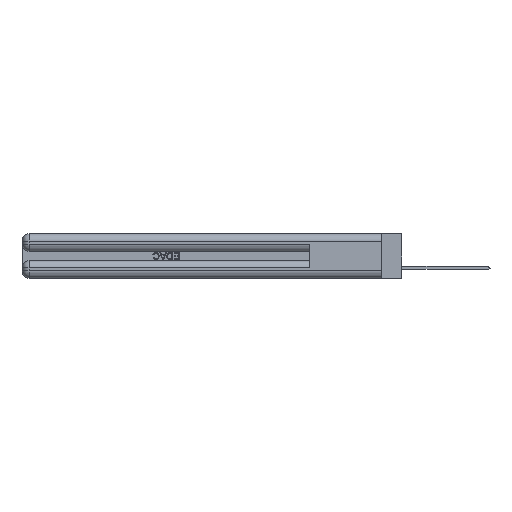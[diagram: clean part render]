
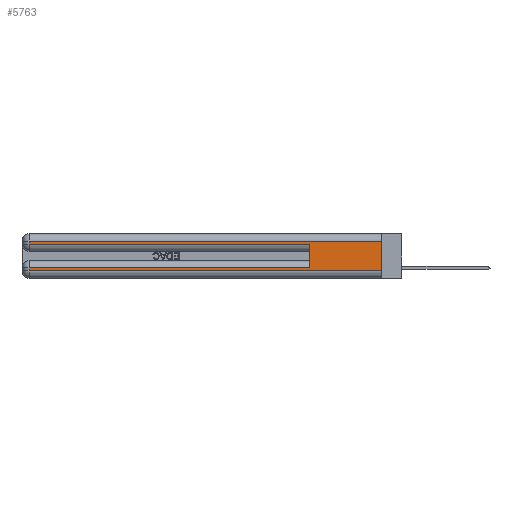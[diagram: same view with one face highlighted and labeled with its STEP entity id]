
A CAD part, left-side view. The second image highlights one B-rep face of the part: STEP entity #5763.
In plain terms, the highlighted planar face has unit normal (-1, 0, 0).
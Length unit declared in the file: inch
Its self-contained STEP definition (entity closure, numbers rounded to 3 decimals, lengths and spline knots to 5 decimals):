
#216 = VERTEX_POINT ( 'NONE', #12801 ) ;
#492 = EDGE_CURVE ( 'NONE', #34399, #29906, #11789, .T. ) ;
#879 = CARTESIAN_POINT ( 'NONE',  ( 0., 0.6, 0.285 ) ) ;
#913 = CARTESIAN_POINT ( 'NONE',  ( 0., 2.94, 0.31 ) ) ;
#2755 = DIRECTION ( 'NONE',  ( 0., 1., 0. ) ) ;
#3484 = DIRECTION ( 'NONE',  ( 0., 0., -1. ) ) ;
#3718 = CARTESIAN_POINT ( 'NONE',  ( 0., 2.94, 0.37 ) ) ;
#3942 = VECTOR ( 'NONE', #3484, 39.37008 ) ;
#4485 = CARTESIAN_POINT ( 'NONE',  ( 0., 0., 0.37 ) ) ;
#4503 = ORIENTED_EDGE ( 'NONE', *, *, #9258, .T. ) ;
#5763 = ADVANCED_FACE ( 'NONE', ( #33104 ), #23446, .F. ) ;
#5998 = EDGE_CURVE ( 'NONE', #10449, #31554, #10714, .T. ) ;
#6727 = DIRECTION ( 'NONE',  ( 0., 0., -1. ) ) ;
#8154 = DIRECTION ( 'NONE',  ( 0., 0., -1. ) ) ;
#8717 = CARTESIAN_POINT ( 'NONE',  ( 0., 2.94, 0.085 ) ) ;
#9068 = EDGE_LOOP ( 'NONE', ( #49584, #4503, #46924, #29225, #31547, #27889, #40500, #33554 ) ) ;
#9258 = EDGE_CURVE ( 'NONE', #47763, #34399, #11208, .T. ) ;
#9619 = CARTESIAN_POINT ( 'NONE',  ( 0., 0., 0.31 ) ) ;
#10283 = EDGE_CURVE ( 'NONE', #216, #36771, #40156, .T. ) ;
#10449 = VERTEX_POINT ( 'NONE', #44480 ) ;
#10714 = LINE ( 'NONE', #11446, #32434 ) ;
#10843 = CARTESIAN_POINT ( 'NONE',  ( 0., 0., 0.37 ) ) ;
#11208 = LINE ( 'NONE', #9619, #26405 ) ;
#11446 = CARTESIAN_POINT ( 'NONE',  ( 0., 0., 0.06 ) ) ;
#11789 = LINE ( 'NONE', #3718, #32353 ) ;
#11893 = CARTESIAN_POINT ( 'NONE',  ( 0., 0., 0.06 ) ) ;
#12801 = CARTESIAN_POINT ( 'NONE',  ( 0., 0.6, 0.085 ) ) ;
#12913 = EDGE_CURVE ( 'NONE', #47763, #31554, #35911, .T. ) ;
#18126 = AXIS2_PLACEMENT_3D ( 'NONE', #4485, #23144, #19394 ) ;
#19277 = DIRECTION ( 'NONE',  ( 0., -1., 0. ) ) ;
#19394 = DIRECTION ( 'NONE',  ( 0., 0., -1. ) ) ;
#23144 = DIRECTION ( 'NONE',  ( 1., 0., 0. ) ) ;
#23446 = PLANE ( 'NONE',  #18126 ) ;
#24958 = CARTESIAN_POINT ( 'NONE',  ( 0., 0., 0.285 ) ) ;
#25082 = DIRECTION ( 'NONE',  ( 0., 0., 1. ) ) ;
#25465 = LINE ( 'NONE', #45061, #45998 ) ;
#26405 = VECTOR ( 'NONE', #37047, 39.37008 ) ;
#26677 = VERTEX_POINT ( 'NONE', #8717 ) ;
#27004 = EDGE_CURVE ( 'NONE', #29906, #36771, #41502, .T. ) ;
#27889 = ORIENTED_EDGE ( 'NONE', *, *, #30357, .T. ) ;
#28816 = DIRECTION ( 'NONE',  ( 0., -1., 0. ) ) ;
#29225 = ORIENTED_EDGE ( 'NONE', *, *, #27004, .T. ) ;
#29587 = CARTESIAN_POINT ( 'NONE',  ( 0., 2.94, 0.285 ) ) ;
#29906 = VERTEX_POINT ( 'NONE', #29587 ) ;
#30357 = EDGE_CURVE ( 'NONE', #216, #26677, #25465, .T. ) ;
#31547 = ORIENTED_EDGE ( 'NONE', *, *, #10283, .F. ) ;
#31554 = VERTEX_POINT ( 'NONE', #11893 ) ;
#32101 = VECTOR ( 'NONE', #6727, 39.37008 ) ;
#32353 = VECTOR ( 'NONE', #8154, 39.37008 ) ;
#32434 = VECTOR ( 'NONE', #19277, 39.37008 ) ;
#33104 = FACE_OUTER_BOUND ( 'NONE', #9068, .T. ) ;
#33554 = ORIENTED_EDGE ( 'NONE', *, *, #5998, .T. ) ;
#34399 = VERTEX_POINT ( 'NONE', #913 ) ;
#35911 = LINE ( 'NONE', #10843, #3942 ) ;
#36393 = CARTESIAN_POINT ( 'NONE',  ( 0., 0.6, 0.145 ) ) ;
#36771 = VERTEX_POINT ( 'NONE', #879 ) ;
#37047 = DIRECTION ( 'NONE',  ( 0., 1., 0. ) ) ;
#37802 = CARTESIAN_POINT ( 'NONE',  ( 0., 2.94, 0.37 ) ) ;
#38822 = LINE ( 'NONE', #37802, #32101 ) ;
#40156 = LINE ( 'NONE', #36393, #42591 ) ;
#40500 = ORIENTED_EDGE ( 'NONE', *, *, #46307, .T. ) ;
#40738 = CARTESIAN_POINT ( 'NONE',  ( 0., 0., 0.31 ) ) ;
#41502 = LINE ( 'NONE', #24958, #46813 ) ;
#42591 = VECTOR ( 'NONE', #25082, 39.37008 ) ;
#44480 = CARTESIAN_POINT ( 'NONE',  ( 0., 2.94, 0.06 ) ) ;
#45061 = CARTESIAN_POINT ( 'NONE',  ( 0., 0., 0.085 ) ) ;
#45998 = VECTOR ( 'NONE', #2755, 39.37008 ) ;
#46307 = EDGE_CURVE ( 'NONE', #26677, #10449, #38822, .T. ) ;
#46813 = VECTOR ( 'NONE', #28816, 39.37008 ) ;
#46924 = ORIENTED_EDGE ( 'NONE', *, *, #492, .T. ) ;
#47763 = VERTEX_POINT ( 'NONE', #40738 ) ;
#49584 = ORIENTED_EDGE ( 'NONE', *, *, #12913, .F. ) ;
